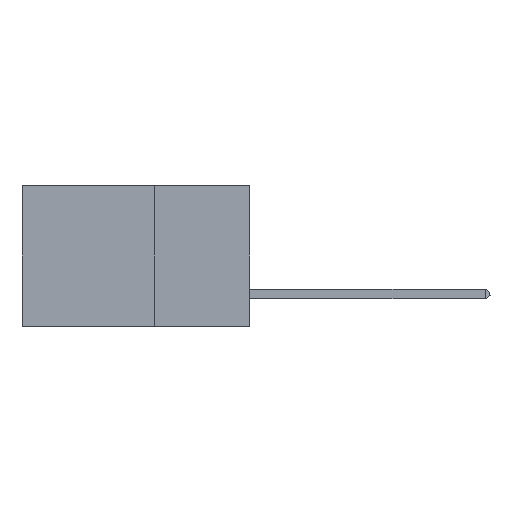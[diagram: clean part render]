
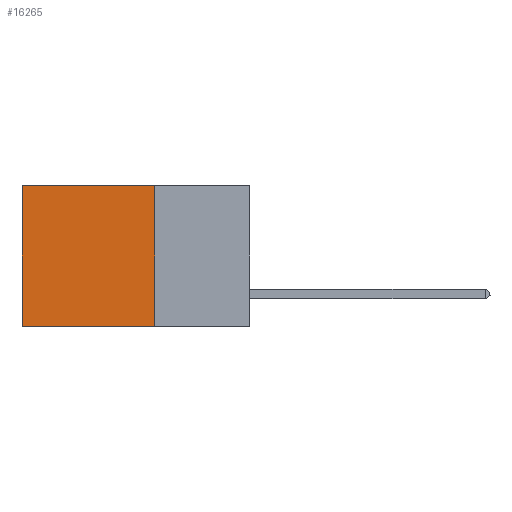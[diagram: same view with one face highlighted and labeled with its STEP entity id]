
A CAD part, left-side view. The second image highlights one B-rep face of the part: STEP entity #16265.
In plain terms, the highlighted planar face has unit normal (-1, 0, 0).
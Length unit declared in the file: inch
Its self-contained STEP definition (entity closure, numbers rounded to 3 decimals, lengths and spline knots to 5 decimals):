
#54 = DIRECTION ( 'NONE',  ( 0., 1., 0. ) ) ;
#221 = EDGE_CURVE ( 'NONE', #5023, #9463, #2506, .T. ) ;
#433 = CARTESIAN_POINT ( 'NONE',  ( 0.2875, 0.25, 0. ) ) ;
#1235 = VERTEX_POINT ( 'NONE', #5492 ) ;
#1393 = CARTESIAN_POINT ( 'NONE',  ( 0.2875, 0.25, -0.37 ) ) ;
#1782 = CARTESIAN_POINT ( 'NONE',  ( 0.2875, 0.25, 0. ) ) ;
#2506 = LINE ( 'NONE', #1782, #7874 ) ;
#3493 = FACE_OUTER_BOUND ( 'NONE', #4397, .T. ) ;
#3551 = VECTOR ( 'NONE', #10209, 39.37008 ) ;
#3924 = VERTEX_POINT ( 'NONE', #10098 ) ;
#3928 = CARTESIAN_POINT ( 'NONE',  ( 0.2875, 0.6, 0. ) ) ;
#4397 = EDGE_LOOP ( 'NONE', ( #6161, #16249, #6263, #11945 ) ) ;
#4832 = LINE ( 'NONE', #16253, #11108 ) ;
#4916 = EDGE_CURVE ( 'NONE', #9463, #3924, #4832, .T. ) ;
#5023 = VERTEX_POINT ( 'NONE', #9861 ) ;
#5492 = CARTESIAN_POINT ( 'NONE',  ( 0.2875, 0.6, 0. ) ) ;
#6161 = ORIENTED_EDGE ( 'NONE', *, *, #7497, .T. ) ;
#6263 = ORIENTED_EDGE ( 'NONE', *, *, #221, .F. ) ;
#7229 = LINE ( 'NONE', #3928, #17786 ) ;
#7497 = EDGE_CURVE ( 'NONE', #1235, #3924, #7229, .T. ) ;
#7874 = VECTOR ( 'NONE', #10398, 39.37008 ) ;
#8585 = DIRECTION ( 'NONE',  ( 1., 0., 0. ) ) ;
#9463 = VERTEX_POINT ( 'NONE', #1393 ) ;
#9861 = CARTESIAN_POINT ( 'NONE',  ( 0.2875, 0.25, 0. ) ) ;
#10098 = CARTESIAN_POINT ( 'NONE',  ( 0.2875, 0.6, -0.37 ) ) ;
#10209 = DIRECTION ( 'NONE',  ( 0., 1., 0. ) ) ;
#10398 = DIRECTION ( 'NONE',  ( 0., 0., -1. ) ) ;
#10734 = LINE ( 'NONE', #17201, #3551 ) ;
#10976 = EDGE_CURVE ( 'NONE', #5023, #1235, #10734, .T. ) ;
#11108 = VECTOR ( 'NONE', #54, 39.37008 ) ;
#11945 = ORIENTED_EDGE ( 'NONE', *, *, #10976, .T. ) ;
#12863 = PLANE ( 'NONE',  #17145 ) ;
#12929 = DIRECTION ( 'NONE',  ( 0., 0., -1. ) ) ;
#14043 = DIRECTION ( 'NONE',  ( 0., 0., -1. ) ) ;
#16249 = ORIENTED_EDGE ( 'NONE', *, *, #4916, .F. ) ;
#16253 = CARTESIAN_POINT ( 'NONE',  ( 0.2875, 0.25, -0.37 ) ) ;
#16265 = ADVANCED_FACE ( 'NONE', ( #3493 ), #12863, .F. ) ;
#17145 = AXIS2_PLACEMENT_3D ( 'NONE', #433, #8585, #12929 ) ;
#17201 = CARTESIAN_POINT ( 'NONE',  ( 0.2875, 0.25, 0. ) ) ;
#17786 = VECTOR ( 'NONE', #14043, 39.37008 ) ;
